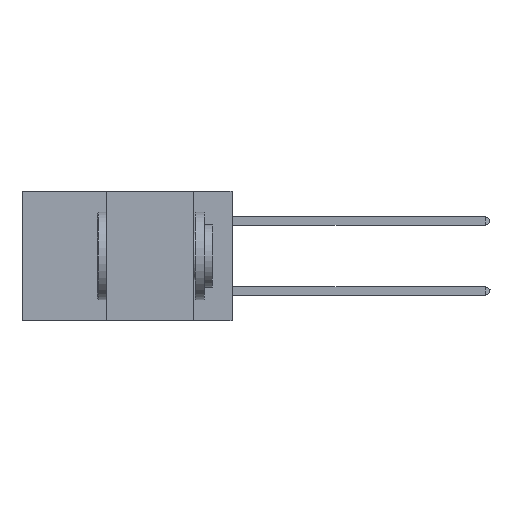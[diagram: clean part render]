
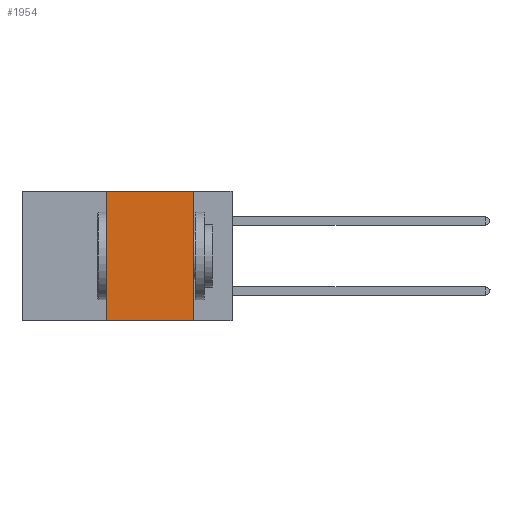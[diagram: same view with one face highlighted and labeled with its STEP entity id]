
A CAD part, left-side view. The second image highlights one B-rep face of the part: STEP entity #1954.
In plain terms, the highlighted planar face has unit normal (-1, 0, 0).
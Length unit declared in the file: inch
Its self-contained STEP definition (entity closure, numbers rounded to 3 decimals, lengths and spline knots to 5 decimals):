
#60 = VECTOR ( 'NONE', #8582, 39.37008 ) ;
#177 = CARTESIAN_POINT ( 'NONE',  ( 0., 0.11, -0.37 ) ) ;
#656 = VECTOR ( 'NONE', #1843, 39.37008 ) ;
#1156 = CARTESIAN_POINT ( 'NONE',  ( 0., 0.36, 0. ) ) ;
#1434 = VECTOR ( 'NONE', #3281, 39.37008 ) ;
#1818 = FACE_OUTER_BOUND ( 'NONE', #5176, .T. ) ;
#1843 = DIRECTION ( 'NONE',  ( 0., -1., 0. ) ) ;
#1954 = ADVANCED_FACE ( 'NONE', ( #1818 ), #7580, .F. ) ;
#2314 = VERTEX_POINT ( 'NONE', #9340 ) ;
#2334 = ORIENTED_EDGE ( 'NONE', *, *, #3183, .F. ) ;
#2796 = LINE ( 'NONE', #5481, #1434 ) ;
#3183 = EDGE_CURVE ( 'NONE', #7482, #4271, #8487, .T. ) ;
#3281 = DIRECTION ( 'NONE',  ( 0., 0., 1. ) ) ;
#3402 = ORIENTED_EDGE ( 'NONE', *, *, #4894, .F. ) ;
#3428 = CARTESIAN_POINT ( 'NONE',  ( 0., 0.11, 0. ) ) ;
#4209 = DIRECTION ( 'NONE',  ( 0., 0., -1. ) ) ;
#4271 = VERTEX_POINT ( 'NONE', #3428 ) ;
#4825 = EDGE_CURVE ( 'NONE', #2314, #7482, #2796, .T. ) ;
#4894 = EDGE_CURVE ( 'NONE', #4271, #6717, #8907, .T. ) ;
#4998 = VECTOR ( 'NONE', #4209, 39.37008 ) ;
#5176 = EDGE_LOOP ( 'NONE', ( #3402, #2334, #8704, #7710 ) ) ;
#5481 = CARTESIAN_POINT ( 'NONE',  ( 0., 0.36, 0. ) ) ;
#5488 = CARTESIAN_POINT ( 'NONE',  ( 0., 0.6, -0.37 ) ) ;
#6084 = AXIS2_PLACEMENT_3D ( 'NONE', #6871, #7641, #8945 ) ;
#6374 = CARTESIAN_POINT ( 'NONE',  ( 0., 0.11, 0. ) ) ;
#6520 = LINE ( 'NONE', #5488, #656 ) ;
#6717 = VERTEX_POINT ( 'NONE', #177 ) ;
#6871 = CARTESIAN_POINT ( 'NONE',  ( 0., 0.6, 0. ) ) ;
#7482 = VERTEX_POINT ( 'NONE', #1156 ) ;
#7551 = EDGE_CURVE ( 'NONE', #2314, #6717, #6520, .T. ) ;
#7580 = PLANE ( 'NONE',  #6084 ) ;
#7641 = DIRECTION ( 'NONE',  ( 1., 0., 0. ) ) ;
#7710 = ORIENTED_EDGE ( 'NONE', *, *, #7551, .T. ) ;
#7852 = CARTESIAN_POINT ( 'NONE',  ( 0., 0.6, 0. ) ) ;
#8487 = LINE ( 'NONE', #7852, #60 ) ;
#8582 = DIRECTION ( 'NONE',  ( 0., -1., 0. ) ) ;
#8704 = ORIENTED_EDGE ( 'NONE', *, *, #4825, .F. ) ;
#8907 = LINE ( 'NONE', #6374, #4998 ) ;
#8945 = DIRECTION ( 'NONE',  ( 0., 0., -1. ) ) ;
#9340 = CARTESIAN_POINT ( 'NONE',  ( 0., 0.36, -0.37 ) ) ;
